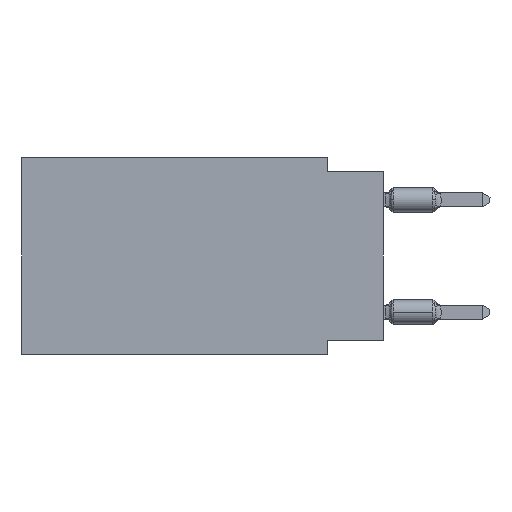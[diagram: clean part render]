
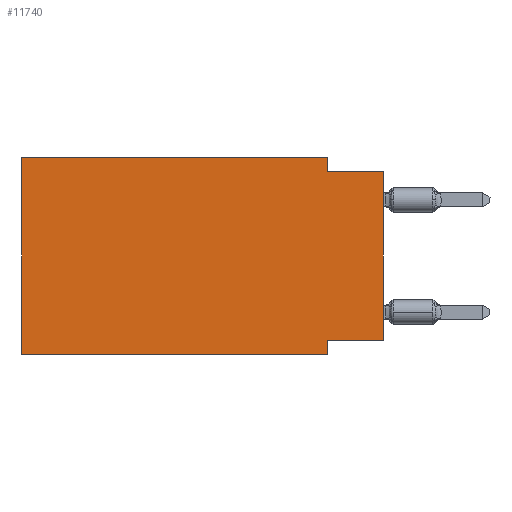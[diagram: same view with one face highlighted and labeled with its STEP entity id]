
A CAD part, left-side view. The second image highlights one B-rep face of the part: STEP entity #11740.
In plain terms, the highlighted planar face has unit normal (-1, 0, 0).
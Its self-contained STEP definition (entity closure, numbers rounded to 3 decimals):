
#314 = AXIS2_PLACEMENT_3D ( 'NONE', #6631, #11749, #7971 ) ;
#710 = LINE ( 'NONE', #11029, #11259 ) ;
#1066 = DIRECTION ( 'NONE',  ( 0., 0., 1. ) ) ;
#1348 = LINE ( 'NONE', #4600, #15953 ) ;
#1707 = DIRECTION ( 'NONE',  ( 0., -1., 0. ) ) ;
#1928 = DIRECTION ( 'NONE',  ( 0., -1., 0. ) ) ;
#1993 = EDGE_CURVE ( 'NONE', #15852, #10828, #4739, .T. ) ;
#2332 = EDGE_LOOP ( 'NONE', ( #4136, #13906, #16336, #10070, #4280, #6155, #16504, #4989 ) ) ;
#2456 = CARTESIAN_POINT ( 'NONE',  ( 0., 16.383, -8.89 ) ) ;
#2727 = CARTESIAN_POINT ( 'NONE',  ( 0., 2.54, 0. ) ) ;
#2829 = VECTOR ( 'NONE', #1066, 1000. ) ;
#2914 = VERTEX_POINT ( 'NONE', #8303 ) ;
#3545 = CARTESIAN_POINT ( 'NONE',  ( 0., 2.54, -8.89 ) ) ;
#3599 = EDGE_CURVE ( 'NONE', #9981, #2914, #14456, .T. ) ;
#4136 = ORIENTED_EDGE ( 'NONE', *, *, #9986, .T. ) ;
#4280 = ORIENTED_EDGE ( 'NONE', *, *, #14915, .F. ) ;
#4584 = VECTOR ( 'NONE', #1928, 1000. ) ;
#4600 = CARTESIAN_POINT ( 'NONE',  ( 0., 0., -8.255 ) ) ;
#4739 = LINE ( 'NONE', #12385, #12528 ) ;
#4989 = ORIENTED_EDGE ( 'NONE', *, *, #14885, .F. ) ;
#5594 = VERTEX_POINT ( 'NONE', #9498 ) ;
#5622 = CARTESIAN_POINT ( 'NONE',  ( 0., 0., -0.635 ) ) ;
#5761 = EDGE_CURVE ( 'NONE', #10828, #5594, #710, .T. ) ;
#5844 = DIRECTION ( 'NONE',  ( 0., -1., 0. ) ) ;
#6155 = ORIENTED_EDGE ( 'NONE', *, *, #3599, .T. ) ;
#6209 = VECTOR ( 'NONE', #8819, 1000. ) ;
#6393 = EDGE_CURVE ( 'NONE', #9701, #2914, #15028, .T. ) ;
#6542 = FACE_OUTER_BOUND ( 'NONE', #2332, .T. ) ;
#6631 = CARTESIAN_POINT ( 'NONE',  ( 0., 16.383, 0. ) ) ;
#6788 = CARTESIAN_POINT ( 'NONE',  ( 0., 16.383, 0. ) ) ;
#7754 = CARTESIAN_POINT ( 'NONE',  ( 0., 2.54, -8.255 ) ) ;
#7971 = DIRECTION ( 'NONE',  ( 0., 0., -1. ) ) ;
#8080 = CARTESIAN_POINT ( 'NONE',  ( 0., 16.383, -8.89 ) ) ;
#8303 = CARTESIAN_POINT ( 'NONE',  ( 0., 2.54, -8.89 ) ) ;
#8650 = DIRECTION ( 'NONE',  ( 0., 0., -1. ) ) ;
#8693 = CARTESIAN_POINT ( 'NONE',  ( 0., 16.383, 0. ) ) ;
#8719 = VERTEX_POINT ( 'NONE', #9726 ) ;
#8819 = DIRECTION ( 'NONE',  ( 0., 0., 1. ) ) ;
#9448 = VERTEX_POINT ( 'NONE', #14564 ) ;
#9498 = CARTESIAN_POINT ( 'NONE',  ( 0., 2.54, -0.635 ) ) ;
#9701 = VERTEX_POINT ( 'NONE', #7754 ) ;
#9726 = CARTESIAN_POINT ( 'NONE',  ( 0., 0., -0.635 ) ) ;
#9981 = VERTEX_POINT ( 'NONE', #2456 ) ;
#9986 = EDGE_CURVE ( 'NONE', #9448, #8719, #15206, .T. ) ;
#10070 = ORIENTED_EDGE ( 'NONE', *, *, #1993, .F. ) ;
#10330 = VECTOR ( 'NONE', #1707, 1000. ) ;
#10828 = VERTEX_POINT ( 'NONE', #2727 ) ;
#11029 = CARTESIAN_POINT ( 'NONE',  ( 0., 2.54, 0. ) ) ;
#11259 = VECTOR ( 'NONE', #13640, 1000. ) ;
#11657 = PLANE ( 'NONE',  #314 ) ;
#11740 = ADVANCED_FACE ( 'NONE', ( #6542 ), #11657, .F. ) ;
#11749 = DIRECTION ( 'NONE',  ( 1., 0., 0. ) ) ;
#12345 = VECTOR ( 'NONE', #8650, 1000. ) ;
#12385 = CARTESIAN_POINT ( 'NONE',  ( 0., 16.383, 0. ) ) ;
#12528 = VECTOR ( 'NONE', #5844, 1000. ) ;
#13059 = EDGE_CURVE ( 'NONE', #5594, #8719, #14435, .T. ) ;
#13581 = LINE ( 'NONE', #8693, #2829 ) ;
#13634 = CARTESIAN_POINT ( 'NONE',  ( 0., 0., 0. ) ) ;
#13640 = DIRECTION ( 'NONE',  ( 0., 0., -1. ) ) ;
#13906 = ORIENTED_EDGE ( 'NONE', *, *, #13059, .F. ) ;
#14435 = LINE ( 'NONE', #5622, #4584 ) ;
#14456 = LINE ( 'NONE', #8080, #10330 ) ;
#14564 = CARTESIAN_POINT ( 'NONE',  ( 0., 0., -8.255 ) ) ;
#14840 = DIRECTION ( 'NONE',  ( 0., 1., 0. ) ) ;
#14885 = EDGE_CURVE ( 'NONE', #9448, #9701, #1348, .T. ) ;
#14915 = EDGE_CURVE ( 'NONE', #9981, #15852, #13581, .T. ) ;
#15028 = LINE ( 'NONE', #3545, #12345 ) ;
#15206 = LINE ( 'NONE', #13634, #6209 ) ;
#15852 = VERTEX_POINT ( 'NONE', #6788 ) ;
#15953 = VECTOR ( 'NONE', #14840, 1000. ) ;
#16336 = ORIENTED_EDGE ( 'NONE', *, *, #5761, .F. ) ;
#16504 = ORIENTED_EDGE ( 'NONE', *, *, #6393, .F. ) ;
